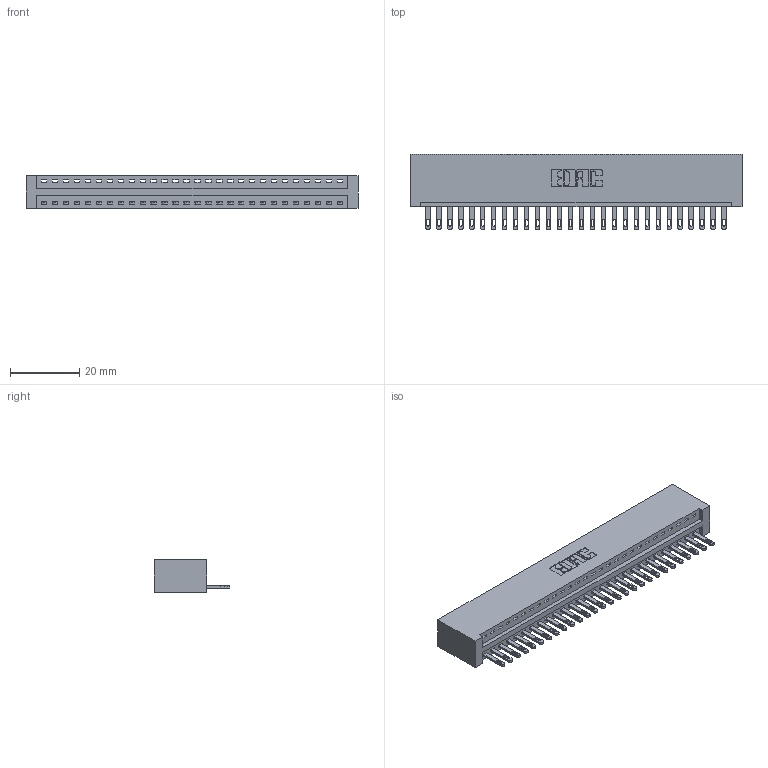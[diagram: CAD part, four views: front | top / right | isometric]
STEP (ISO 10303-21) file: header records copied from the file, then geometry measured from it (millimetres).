
FILE_DESCRIPTION (( 'STEP AP203' ), '1' );
FILE_NAME ('896-028-500-101.STEP', '2021-07-27T18:13:17', ( '' ), ( '' ), 'SwSTEP 2.0', 'SolidWorks 2020', '' );
FILE_SCHEMA (( 'CONFIG_CONTROL_DESIGN' ));
Length unit declared in the file: inch
Products named in the file (3): 846 Part_No Mounting Lugs; 345-292-001_345-293-100; 896-028-500-101
Assembly tree (29 placements, depth 2):
  896-028-500-101
    846 Part_No Mounting Lugs
    345-292-001_345-293-100  x28
Bounding box: 96.14 x 21.84 x 9.4 mm (x, y, z)
Volume: 9672.9 mm3; surface area: 12079.2 mm2
Topology: 29 solids, 29 shells, 1626 faces, 5009 edges, 3338 vertices
Faces by surface type: plane 1024, cylinder 602
Entity records: 18915 total; most frequent: CARTESIAN_POINT 3252, ORIENTED_EDGE 3214, DIRECTION 2883, EDGE_CURVE 1607, LINE 1367, VECTOR 1367, VERTEX_POINT 1070, AXIS2_PLACEMENT_3D 758
